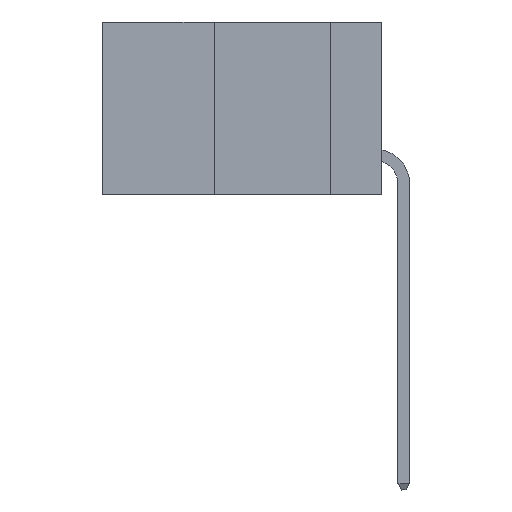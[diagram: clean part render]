
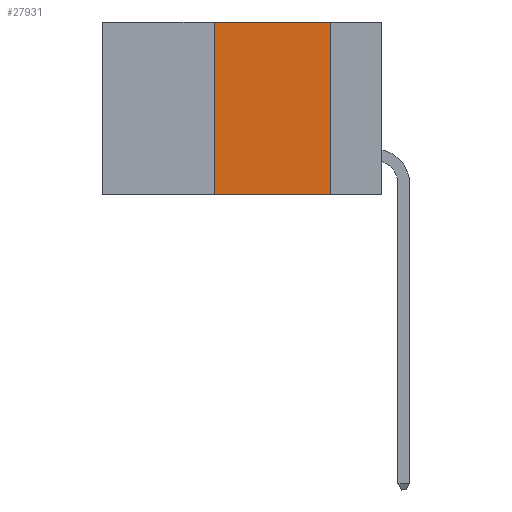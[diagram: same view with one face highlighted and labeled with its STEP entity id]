
A CAD part, left-side view. The second image highlights one B-rep face of the part: STEP entity #27931.
In plain terms, the highlighted planar face has unit normal (-1, 0, 0).
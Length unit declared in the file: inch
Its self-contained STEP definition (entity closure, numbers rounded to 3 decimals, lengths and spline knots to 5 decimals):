
#411 = EDGE_CURVE ( 'NONE', #28369, #37853, #30122, .T. ) ;
#758 = VERTEX_POINT ( 'NONE', #4363 ) ;
#2033 = DIRECTION ( 'NONE',  ( 0., 0., -1. ) ) ;
#2490 = EDGE_CURVE ( 'NONE', #35552, #37853, #22205, .T. ) ;
#3181 = ORIENTED_EDGE ( 'NONE', *, *, #411, .T. ) ;
#3780 = DIRECTION ( 'NONE',  ( 0., -1., 0. ) ) ;
#4353 = CARTESIAN_POINT ( 'NONE',  ( 0., 0.6, 0. ) ) ;
#4363 = CARTESIAN_POINT ( 'NONE',  ( 0., 0.36, 0. ) ) ;
#4819 = EDGE_LOOP ( 'NONE', ( #14114, #8111, #29803, #3181 ) ) ;
#8111 = ORIENTED_EDGE ( 'NONE', *, *, #27621, .F. ) ;
#10604 = CARTESIAN_POINT ( 'NONE',  ( 0., 0.6, -0.37 ) ) ;
#12698 = DIRECTION ( 'NONE',  ( 0., 0., 1. ) ) ;
#14114 = ORIENTED_EDGE ( 'NONE', *, *, #2490, .F. ) ;
#17037 = VECTOR ( 'NONE', #3780, 39.37008 ) ;
#17893 = VECTOR ( 'NONE', #2033, 39.37008 ) ;
#20879 = CARTESIAN_POINT ( 'NONE',  ( 0., 0.6, 0. ) ) ;
#22205 = LINE ( 'NONE', #28760, #17893 ) ;
#23090 = LINE ( 'NONE', #29721, #37648 ) ;
#24635 = DIRECTION ( 'NONE',  ( 0., -1., 0. ) ) ;
#25238 = VECTOR ( 'NONE', #24635, 39.37008 ) ;
#26735 = EDGE_CURVE ( 'NONE', #28369, #758, #23090, .T. ) ;
#27238 = FACE_OUTER_BOUND ( 'NONE', #4819, .T. ) ;
#27621 = EDGE_CURVE ( 'NONE', #758, #35552, #34850, .T. ) ;
#27931 = ADVANCED_FACE ( 'NONE', ( #27238 ), #42274, .F. ) ;
#28369 = VERTEX_POINT ( 'NONE', #32287 ) ;
#28760 = CARTESIAN_POINT ( 'NONE',  ( 0., 0.11, 0. ) ) ;
#29124 = DIRECTION ( 'NONE',  ( 0., 0., -1. ) ) ;
#29721 = CARTESIAN_POINT ( 'NONE',  ( 0., 0.36, 0. ) ) ;
#29803 = ORIENTED_EDGE ( 'NONE', *, *, #26735, .F. ) ;
#30122 = LINE ( 'NONE', #10604, #25238 ) ;
#32287 = CARTESIAN_POINT ( 'NONE',  ( 0., 0.36, -0.37 ) ) ;
#32553 = AXIS2_PLACEMENT_3D ( 'NONE', #4353, #36234, #29124 ) ;
#34850 = LINE ( 'NONE', #20879, #17037 ) ;
#35552 = VERTEX_POINT ( 'NONE', #37070 ) ;
#36234 = DIRECTION ( 'NONE',  ( 1., 0., 0. ) ) ;
#37070 = CARTESIAN_POINT ( 'NONE',  ( 0., 0.11, 0. ) ) ;
#37648 = VECTOR ( 'NONE', #12698, 39.37008 ) ;
#37853 = VERTEX_POINT ( 'NONE', #44825 ) ;
#42274 = PLANE ( 'NONE',  #32553 ) ;
#44825 = CARTESIAN_POINT ( 'NONE',  ( 0., 0.11, -0.37 ) ) ;
